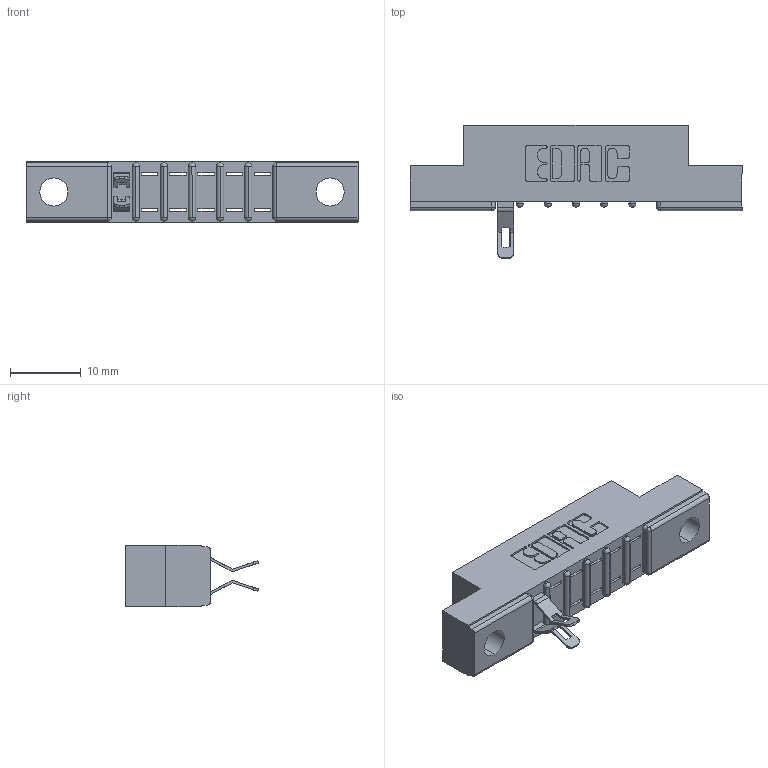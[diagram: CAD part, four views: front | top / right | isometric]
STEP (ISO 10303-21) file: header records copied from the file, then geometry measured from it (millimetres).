
FILE_DESCRIPTION (( 'STEP AP203' ), '1' );
FILE_NAME ('307-012-555-202.STEP', '2018-08-02T23:13:41', ( '' ), ( '' ), 'SwSTEP 2.0', 'SolidWorks 2016', '' );
FILE_SCHEMA (( 'CONFIG_CONTROL_DESIGN' ));
Length unit declared in the file: inch
Products named in the file (3): 307 Part_.128 Dia Mounting Holes; 307-290-001_555; 307-012-555-202
Assembly tree (3 placements, depth 2):
  307-012-555-202
    307 Part_.128 Dia Mounting Holes
    307-290-001_555  x2
Bounding box: 46.79 x 18.75 x 8.71 mm (x, y, z)
Volume: 2850.8 mm3; surface area: 3315.9 mm2
Topology: 3 solids, 3 shells, 347 faces, 1005 edges, 646 vertices
Faces by surface type: plane 198, cylinder 135, sphere 14
Entity records: 9993 total; most frequent: CARTESIAN_POINT 1692, ORIENTED_EDGE 1684, DIRECTION 1670, EDGE_CURVE 842, LINE 618, VECTOR 618, VERTEX_POINT 548, AXIS2_PLACEMENT_3D 526
